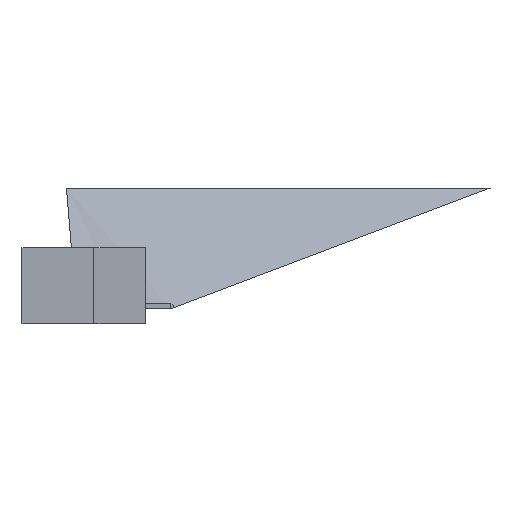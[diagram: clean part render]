
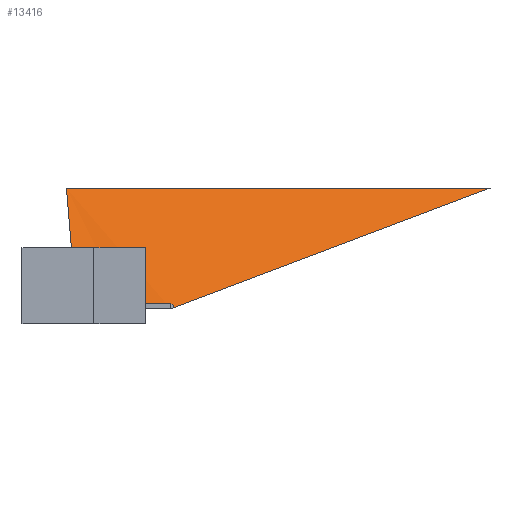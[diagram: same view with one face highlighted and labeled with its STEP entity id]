
A CAD part, left-side view. The second image highlights one B-rep face of the part: STEP entity #13416.
In plain terms, the highlighted face is planar.
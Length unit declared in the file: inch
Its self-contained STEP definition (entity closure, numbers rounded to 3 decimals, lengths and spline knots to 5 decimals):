
#153 = DIRECTION ( 'NONE',  ( 0., 0., 1. ) ) ;
#186 = CIRCLE ( 'NONE', #16354, 0.006 ) ;
#189 = CARTESIAN_POINT ( 'NONE',  ( 0.33619, 0.0125, -0.025 ) ) ;
#234 = EDGE_CURVE ( 'NONE', #11870, #11946, #7792, .T. ) ;
#855 = EDGE_CURVE ( 'NONE', #10141, #2375, #3208, .T. ) ;
#976 = ORIENTED_EDGE ( 'NONE', *, *, #4473, .F. ) ;
#1048 = ORIENTED_EDGE ( 'NONE', *, *, #12061, .F. ) ;
#1204 = EDGE_CURVE ( 'NONE', #11870, #10727, #1274, .T. ) ;
#1274 = LINE ( 'NONE', #10869, #14296 ) ;
#1290 = DIRECTION ( 'NONE',  ( 1., 0., 0. ) ) ;
#1314 = LINE ( 'NONE', #12505, #14730 ) ;
#1349 = LINE ( 'NONE', #16179, #8037 ) ;
#1353 = DIRECTION ( 'NONE',  ( -0.928, 0., -0.373 ) ) ;
#1424 = DIRECTION ( 'NONE',  ( 1., 0., 0. ) ) ;
#2120 = ORIENTED_EDGE ( 'NONE', *, *, #10119, .T. ) ;
#2367 = CARTESIAN_POINT ( 'NONE',  ( 0., 0.6, -0.37 ) ) ;
#2375 = VERTEX_POINT ( 'NONE', #16579 ) ;
#2382 = CARTESIAN_POINT ( 'NONE',  ( 0.58021, 0.0125, -0.025 ) ) ;
#2658 = CARTESIAN_POINT ( 'NONE',  ( 0.58021, 0.0125, -0.025 ) ) ;
#2842 = DIRECTION ( 'NONE',  ( 1., 0., 0. ) ) ;
#3015 = EDGE_CURVE ( 'NONE', #7294, #10517, #4952, .T. ) ;
#3078 = CARTESIAN_POINT ( 'NONE',  ( 0.61321, 0.0125, 0.0125 ) ) ;
#3208 = LINE ( 'NONE', #3078, #7143 ) ;
#3644 = CARTESIAN_POINT ( 'NONE',  ( 0.61321, 0.0125, -0.0225 ) ) ;
#3683 = CARTESIAN_POINT ( 'NONE',  ( 0.34621, 0.0125, 0.006 ) ) ;
#3890 = CARTESIAN_POINT ( 'NONE',  ( 2.3475, 0.6, -0.37 ) ) ;
#4473 = EDGE_CURVE ( 'NONE', #8556, #10141, #6468, .T. ) ;
#4852 = CARTESIAN_POINT ( 'NONE',  ( 0.33619, 0.0125, -0.006 ) ) ;
#4858 = DIRECTION ( 'NONE',  ( -1., 0., 0. ) ) ;
#4876 = EDGE_CURVE ( 'NONE', #8085, #8930, #6859, .T. ) ;
#4938 = DIRECTION ( 'NONE',  ( 1., 0., 0. ) ) ;
#4952 = CIRCLE ( 'NONE', #14172, 0.006 ) ;
#4984 = AXIS2_PLACEMENT_3D ( 'NONE', #189, #14620, #6989 ) ;
#5139 = CARTESIAN_POINT ( 'NONE',  ( 0.33619, 0.0125, -0.025 ) ) ;
#5655 = PLANE ( 'NONE',  #4984 ) ;
#5788 = DIRECTION ( 'NONE',  ( 0., 0., -1. ) ) ;
#6030 = VERTEX_POINT ( 'NONE', #6472 ) ;
#6355 = VECTOR ( 'NONE', #153, 39.37008 ) ;
#6468 = CIRCLE ( 'NONE', #10117, 0.01 ) ;
#6472 = CARTESIAN_POINT ( 'NONE',  ( 0.34621, 0.0125, -0.006 ) ) ;
#6606 = DIRECTION ( 'NONE',  ( 0., 0., -1. ) ) ;
#6624 = EDGE_CURVE ( 'NONE', #7639, #12397, #14196, .T. ) ;
#6645 = CARTESIAN_POINT ( 'NONE',  ( 0.33619, 0.0125, 0.025 ) ) ;
#6650 = ORIENTED_EDGE ( 'NONE', *, *, #855, .F. ) ;
#6684 = VERTEX_POINT ( 'NONE', #2382 ) ;
#6859 = LINE ( 'NONE', #2367, #13254 ) ;
#6989 = DIRECTION ( 'NONE',  ( 1., 0., 0. ) ) ;
#7080 = CARTESIAN_POINT ( 'NONE',  ( 0.79521, 0.0125, -0.0125 ) ) ;
#7143 = VECTOR ( 'NONE', #2842, 39.37008 ) ;
#7153 = EDGE_CURVE ( 'NONE', #11946, #8556, #1349, .T. ) ;
#7291 = CARTESIAN_POINT ( 'NONE',  ( 0.61321, 0.0125, -0.0125 ) ) ;
#7294 = VERTEX_POINT ( 'NONE', #3683 ) ;
#7448 = DIRECTION ( 'NONE',  ( 0., 1., 0. ) ) ;
#7474 = EDGE_CURVE ( 'NONE', #12397, #6684, #14165, .T. ) ;
#7639 = VERTEX_POINT ( 'NONE', #12094 ) ;
#7792 = LINE ( 'NONE', #6645, #8215 ) ;
#7841 = DIRECTION ( 'NONE',  ( 0., -1., 0. ) ) ;
#7922 = CARTESIAN_POINT ( 'NONE',  ( 0.33619, 0.0125, -0.025 ) ) ;
#8037 = VECTOR ( 'NONE', #13717, 39.37008 ) ;
#8085 = VERTEX_POINT ( 'NONE', #3890 ) ;
#8102 = CARTESIAN_POINT ( 'NONE',  ( 0.33619, 0.0125, 0.006 ) ) ;
#8211 = LINE ( 'NONE', #14734, #11588 ) ;
#8215 = VECTOR ( 'NONE', #1290, 39.37008 ) ;
#8234 = CARTESIAN_POINT ( 'NONE',  ( 0.61321, 0.0125, 0.0125 ) ) ;
#8376 = EDGE_CURVE ( 'NONE', #11551, #13246, #8211, .T. ) ;
#8467 = EDGE_CURVE ( 'NONE', #10517, #6030, #186, .T. ) ;
#8556 = VERTEX_POINT ( 'NONE', #11443 ) ;
#8726 = AXIS2_PLACEMENT_3D ( 'NONE', #3644, #12672, #4938 ) ;
#8860 = CARTESIAN_POINT ( 'NONE',  ( 0.60948, 0.0125, -0.01322 ) ) ;
#8930 = VERTEX_POINT ( 'NONE', #13456 ) ;
#9034 = EDGE_LOOP ( 'NONE', ( #9279, #9293, #9941, #12258, #10604, #12242, #9424, #13273, #10188, #1048, #2120, #6650, #976, #14616, #13107 ) ) ;
#9279 = ORIENTED_EDGE ( 'NONE', *, *, #1204, .T. ) ;
#9293 = ORIENTED_EDGE ( 'NONE', *, *, #4876, .T. ) ;
#9413 = LINE ( 'NONE', #7291, #15632 ) ;
#9424 = ORIENTED_EDGE ( 'NONE', *, *, #15719, .T. ) ;
#9666 = DIRECTION ( 'NONE',  ( 1., 0., 0. ) ) ;
#9767 = FACE_OUTER_BOUND ( 'NONE', #9034, .T. ) ;
#9874 = DIRECTION ( 'NONE',  ( 0., 1., 0. ) ) ;
#9941 = ORIENTED_EDGE ( 'NONE', *, *, #3015, .T. ) ;
#10117 = AXIS2_PLACEMENT_3D ( 'NONE', #16603, #7841, #1424 ) ;
#10119 = EDGE_CURVE ( 'NONE', #15340, #2375, #16431, .T. ) ;
#10141 = VERTEX_POINT ( 'NONE', #8234 ) ;
#10188 = ORIENTED_EDGE ( 'NONE', *, *, #6624, .F. ) ;
#10459 = EDGE_CURVE ( 'NONE', #6030, #11551, #1314, .T. ) ;
#10467 = DIRECTION ( 'NONE',  ( 1., 0., 0. ) ) ;
#10517 = VERTEX_POINT ( 'NONE', #12684 ) ;
#10604 = ORIENTED_EDGE ( 'NONE', *, *, #10459, .T. ) ;
#10727 = VERTEX_POINT ( 'NONE', #8102 ) ;
#10789 = CARTESIAN_POINT ( 'NONE',  ( 0.79521, 0.0125, -0.025 ) ) ;
#10849 = CARTESIAN_POINT ( 'NONE',  ( 0.33619, 0.0125, 0.025 ) ) ;
#10869 = CARTESIAN_POINT ( 'NONE',  ( 0.33619, 0.0125, -0.025 ) ) ;
#11205 = DIRECTION ( 'NONE',  ( -1., 0., 0. ) ) ;
#11443 = CARTESIAN_POINT ( 'NONE',  ( 0.60948, 0.0125, 0.01322 ) ) ;
#11551 = VERTEX_POINT ( 'NONE', #4852 ) ;
#11588 = VECTOR ( 'NONE', #5788, 39.37008 ) ;
#11870 = VERTEX_POINT ( 'NONE', #10849 ) ;
#11946 = VERTEX_POINT ( 'NONE', #15902 ) ;
#12061 = EDGE_CURVE ( 'NONE', #15340, #7639, #9413, .T. ) ;
#12094 = CARTESIAN_POINT ( 'NONE',  ( 0.61321, 0.0125, -0.0125 ) ) ;
#12242 = ORIENTED_EDGE ( 'NONE', *, *, #8376, .T. ) ;
#12258 = ORIENTED_EDGE ( 'NONE', *, *, #8467, .T. ) ;
#12397 = VERTEX_POINT ( 'NONE', #8860 ) ;
#12407 = CARTESIAN_POINT ( 'NONE',  ( 0.34621, 0.0125, 0. ) ) ;
#12505 = CARTESIAN_POINT ( 'NONE',  ( 0.33619, 0.0125, -0.006 ) ) ;
#12672 = DIRECTION ( 'NONE',  ( 0., -1., 0. ) ) ;
#12684 = CARTESIAN_POINT ( 'NONE',  ( 0.35221, 0.0125, 0. ) ) ;
#13107 = ORIENTED_EDGE ( 'NONE', *, *, #234, .F. ) ;
#13246 = VERTEX_POINT ( 'NONE', #7922 ) ;
#13254 = VECTOR ( 'NONE', #4858, 39.37008 ) ;
#13273 = ORIENTED_EDGE ( 'NONE', *, *, #7474, .F. ) ;
#13416 = ADVANCED_FACE ( 'NONE', ( #9767 ), #5655, .T. ) ;
#13456 = CARTESIAN_POINT ( 'NONE',  ( 0.2875, 0.6, -0.37 ) ) ;
#13717 = DIRECTION ( 'NONE',  ( 0.928, 0., -0.373 ) ) ;
#13766 = VECTOR ( 'NONE', #1353, 39.37008 ) ;
#13849 = DIRECTION ( 'NONE',  ( -1., 0., 0. ) ) ;
#13968 = LINE ( 'NONE', #5139, #16457 ) ;
#14165 = LINE ( 'NONE', #2658, #13766 ) ;
#14172 = AXIS2_PLACEMENT_3D ( 'NONE', #12407, #9874, #9666 ) ;
#14196 = CIRCLE ( 'NONE', #8726, 0.01 ) ;
#14296 = VECTOR ( 'NONE', #6606, 39.37008 ) ;
#14616 = ORIENTED_EDGE ( 'NONE', *, *, #7153, .F. ) ;
#14620 = DIRECTION ( 'NONE',  ( 0., -1., 0. ) ) ;
#14730 = VECTOR ( 'NONE', #13849, 39.37008 ) ;
#14734 = CARTESIAN_POINT ( 'NONE',  ( 0.33619, 0.0125, -0.025 ) ) ;
#15048 = CARTESIAN_POINT ( 'NONE',  ( 0.34621, 0.0125, 0. ) ) ;
#15340 = VERTEX_POINT ( 'NONE', #7080 ) ;
#15632 = VECTOR ( 'NONE', #11205, 39.37008 ) ;
#15719 = EDGE_CURVE ( 'NONE', #13246, #6684, #13968, .T. ) ;
#15902 = CARTESIAN_POINT ( 'NONE',  ( 0.58021, 0.0125, 0.025 ) ) ;
#16179 = CARTESIAN_POINT ( 'NONE',  ( 0.58021, 0.0125, 0.025 ) ) ;
#16244 = DIRECTION ( 'NONE',  ( 1., 0., 0. ) ) ;
#16354 = AXIS2_PLACEMENT_3D ( 'NONE', #15048, #7448, #16244 ) ;
#16431 = LINE ( 'NONE', #10789, #6355 ) ;
#16457 = VECTOR ( 'NONE', #10467, 39.37008 ) ;
#16579 = CARTESIAN_POINT ( 'NONE',  ( 0.79521, 0.0125, 0.0125 ) ) ;
#16603 = CARTESIAN_POINT ( 'NONE',  ( 0.61321, 0.0125, 0.0225 ) ) ;
